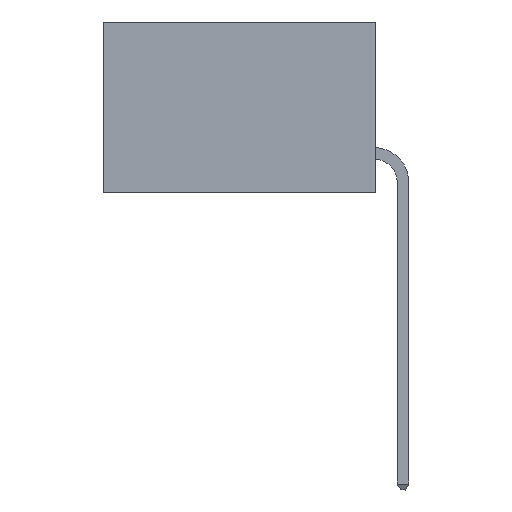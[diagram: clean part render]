
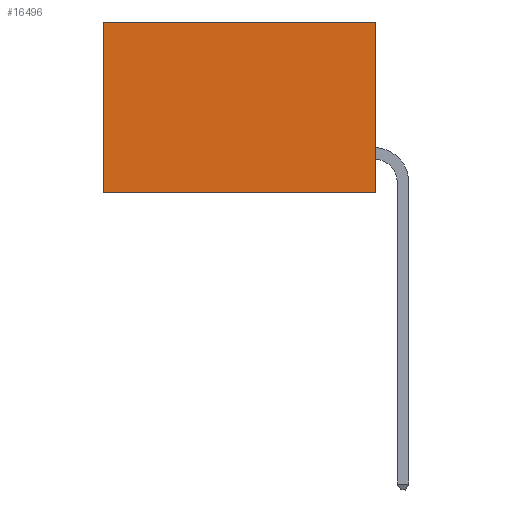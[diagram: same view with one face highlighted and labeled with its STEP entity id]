
A CAD part, left-side view. The second image highlights one B-rep face of the part: STEP entity #16496.
In plain terms, the highlighted planar face has unit normal (-1, 0, 0).
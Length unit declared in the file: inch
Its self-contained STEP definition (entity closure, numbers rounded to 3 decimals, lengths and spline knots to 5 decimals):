
#1212 = LINE ( 'NONE', #7143, #15624 ) ;
#1341 = VERTEX_POINT ( 'NONE', #2694 ) ;
#1485 = CARTESIAN_POINT ( 'NONE',  ( 0.277, 0.59, -0.37 ) ) ;
#2038 = EDGE_CURVE ( 'NONE', #14540, #17213, #1212, .T. ) ;
#2694 = CARTESIAN_POINT ( 'NONE',  ( 0.277, 0., -0.37 ) ) ;
#4443 = EDGE_CURVE ( 'NONE', #14540, #1341, #15112, .T. ) ;
#4595 = ORIENTED_EDGE ( 'NONE', *, *, #10196, .T. ) ;
#4596 = VECTOR ( 'NONE', #7958, 39.37008 ) ;
#4666 = CARTESIAN_POINT ( 'NONE',  ( 0.277, 0.59, 0. ) ) ;
#5067 = ORIENTED_EDGE ( 'NONE', *, *, #8327, .F. ) ;
#5975 = PLANE ( 'NONE',  #6093 ) ;
#6093 = AXIS2_PLACEMENT_3D ( 'NONE', #15873, #7431, #17237 ) ;
#6468 = VERTEX_POINT ( 'NONE', #12573 ) ;
#7143 = CARTESIAN_POINT ( 'NONE',  ( 0.277, 0., 0. ) ) ;
#7431 = DIRECTION ( 'NONE',  ( 1., 0., 0. ) ) ;
#7958 = DIRECTION ( 'NONE',  ( 0., 1., 0. ) ) ;
#7964 = CARTESIAN_POINT ( 'NONE',  ( 0.277, 0., 0. ) ) ;
#8161 = CARTESIAN_POINT ( 'NONE',  ( 0.277, 0., -0.37 ) ) ;
#8327 = EDGE_CURVE ( 'NONE', #1341, #6468, #8899, .T. ) ;
#8899 = LINE ( 'NONE', #8161, #4596 ) ;
#9280 = DIRECTION ( 'NONE',  ( 0., 1., 0. ) ) ;
#9820 = ORIENTED_EDGE ( 'NONE', *, *, #2038, .T. ) ;
#10196 = EDGE_CURVE ( 'NONE', #17213, #6468, #14792, .T. ) ;
#11669 = DIRECTION ( 'NONE',  ( 0., 0., -1. ) ) ;
#12573 = CARTESIAN_POINT ( 'NONE',  ( 0.277, 0.59, -0.37 ) ) ;
#12964 = DIRECTION ( 'NONE',  ( 0., 0., -1. ) ) ;
#13475 = CARTESIAN_POINT ( 'NONE',  ( 0.277, 0., -0.37 ) ) ;
#13765 = FACE_OUTER_BOUND ( 'NONE', #15998, .T. ) ;
#14540 = VERTEX_POINT ( 'NONE', #7964 ) ;
#14792 = LINE ( 'NONE', #1485, #18418 ) ;
#15112 = LINE ( 'NONE', #13475, #18314 ) ;
#15624 = VECTOR ( 'NONE', #9280, 39.37008 ) ;
#15873 = CARTESIAN_POINT ( 'NONE',  ( 0.277, 0., -0.37 ) ) ;
#15998 = EDGE_LOOP ( 'NONE', ( #4595, #5067, #16361, #9820 ) ) ;
#16361 = ORIENTED_EDGE ( 'NONE', *, *, #4443, .F. ) ;
#16496 = ADVANCED_FACE ( 'NONE', ( #13765 ), #5975, .F. ) ;
#17213 = VERTEX_POINT ( 'NONE', #4666 ) ;
#17237 = DIRECTION ( 'NONE',  ( 0., 0., -1. ) ) ;
#18314 = VECTOR ( 'NONE', #12964, 39.37008 ) ;
#18418 = VECTOR ( 'NONE', #11669, 39.37008 ) ;
